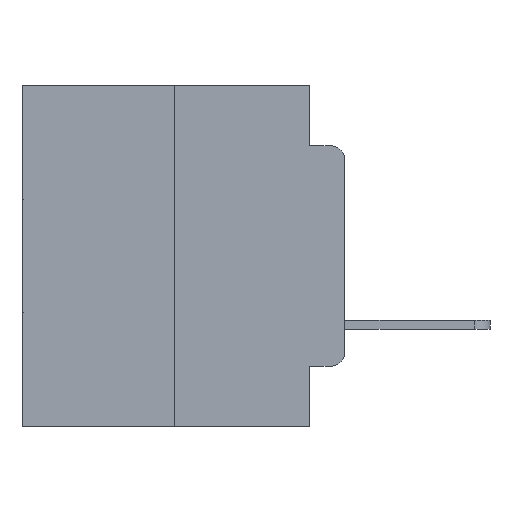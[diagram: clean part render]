
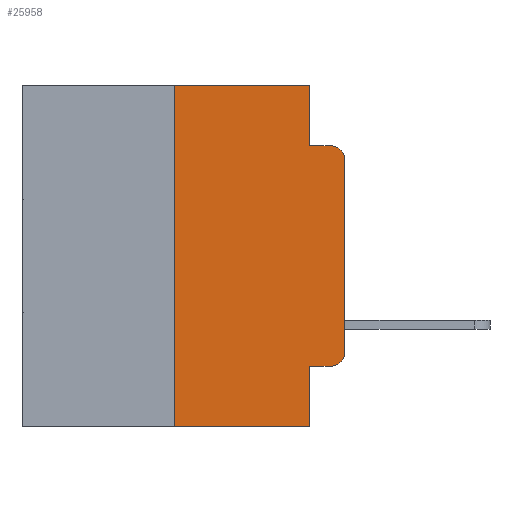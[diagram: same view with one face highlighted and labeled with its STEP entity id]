
A CAD part, left-side view. The second image highlights one B-rep face of the part: STEP entity #25958.
In plain terms, the highlighted planar face has unit normal (-1, 0, 0).
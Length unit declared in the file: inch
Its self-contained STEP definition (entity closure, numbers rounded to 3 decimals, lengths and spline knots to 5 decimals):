
#307 = EDGE_CURVE ( 'NONE', #18999, #11855, #12289, .T. ) ;
#1057 = DIRECTION ( 'NONE',  ( 0., 0., 1. ) ) ;
#2046 = EDGE_CURVE ( 'NONE', #11855, #27441, #28759, .T. ) ;
#3486 = ORIENTED_EDGE ( 'NONE', *, *, #28322, .T. ) ;
#3805 = CARTESIAN_POINT ( 'NONE',  ( 0., 0.473, 0. ) ) ;
#3833 = VERTEX_POINT ( 'NONE', #8795 ) ;
#4408 = LINE ( 'NONE', #28367, #21499 ) ;
#4472 = DIRECTION ( 'NONE',  ( 0., 0., -1. ) ) ;
#4509 = CIRCLE ( 'NONE', #9786, 0.02 ) ;
#4801 = ORIENTED_EDGE ( 'NONE', *, *, #6976, .T. ) ;
#5024 = CARTESIAN_POINT ( 'NONE',  ( 0., 0.25, 0. ) ) ;
#5761 = DIRECTION ( 'NONE',  ( -1., 0., 0. ) ) ;
#6005 = DIRECTION ( 'NONE',  ( 0., 0., -1. ) ) ;
#6073 = CARTESIAN_POINT ( 'NONE',  ( 0., 0.02, -0.3915 ) ) ;
#6218 = LINE ( 'NONE', #12638, #6965 ) ;
#6262 = VECTOR ( 'NONE', #6005, 39.37008 ) ;
#6522 = ORIENTED_EDGE ( 'NONE', *, *, #20888, .T. ) ;
#6965 = VECTOR ( 'NONE', #25672, 39.37008 ) ;
#6976 = EDGE_CURVE ( 'NONE', #25362, #27441, #17237, .T. ) ;
#7491 = FACE_OUTER_BOUND ( 'NONE', #21758, .T. ) ;
#7648 = VERTEX_POINT ( 'NONE', #16411 ) ;
#8306 = CARTESIAN_POINT ( 'NONE',  ( 0., 0.051, 0. ) ) ;
#8373 = DIRECTION ( 'NONE',  ( 0., 0., -1. ) ) ;
#8466 = EDGE_CURVE ( 'NONE', #13363, #25362, #14422, .T. ) ;
#8471 = VECTOR ( 'NONE', #1057, 39.37008 ) ;
#8795 = CARTESIAN_POINT ( 'NONE',  ( 0., 0.25, -0.5 ) ) ;
#8812 = ORIENTED_EDGE ( 'NONE', *, *, #13742, .F. ) ;
#9038 = CARTESIAN_POINT ( 'NONE',  ( 0., 0., -0.1085 ) ) ;
#9478 = VECTOR ( 'NONE', #16939, 39.37008 ) ;
#9786 = AXIS2_PLACEMENT_3D ( 'NONE', #6073, #21584, #8373 ) ;
#11038 = CARTESIAN_POINT ( 'NONE',  ( 0., 0.02, -0.4115 ) ) ;
#11855 = VERTEX_POINT ( 'NONE', #20120 ) ;
#12009 = CARTESIAN_POINT ( 'NONE',  ( 0., 0.02, -0.0885 ) ) ;
#12289 = LINE ( 'NONE', #8306, #6262 ) ;
#12303 = ORIENTED_EDGE ( 'NONE', *, *, #2046, .F. ) ;
#12527 = DIRECTION ( 'NONE',  ( 0., -1., 0. ) ) ;
#12638 = CARTESIAN_POINT ( 'NONE',  ( 0., 0.051, 0. ) ) ;
#12788 = ORIENTED_EDGE ( 'NONE', *, *, #27973, .F. ) ;
#13208 = VERTEX_POINT ( 'NONE', #22262 ) ;
#13363 = VERTEX_POINT ( 'NONE', #24741 ) ;
#13496 = CARTESIAN_POINT ( 'NONE',  ( 0., 0.473, 0. ) ) ;
#13694 = DIRECTION ( 'NONE',  ( 0., 0., 1. ) ) ;
#13742 = EDGE_CURVE ( 'NONE', #22176, #18999, #16349, .T. ) ;
#13881 = ORIENTED_EDGE ( 'NONE', *, *, #22297, .F. ) ;
#14422 = LINE ( 'NONE', #19356, #8471 ) ;
#15619 = ORIENTED_EDGE ( 'NONE', *, *, #8466, .T. ) ;
#15647 = VECTOR ( 'NONE', #21687, 39.37008 ) ;
#16349 = LINE ( 'NONE', #3805, #15647 ) ;
#16411 = CARTESIAN_POINT ( 'NONE',  ( 0., 0.051, -0.5 ) ) ;
#16425 = VECTOR ( 'NONE', #13694, 39.37008 ) ;
#16939 = DIRECTION ( 'NONE',  ( 0., -1., 0. ) ) ;
#16985 = CARTESIAN_POINT ( 'NONE',  ( 0., 0.051, 0. ) ) ;
#17038 = CARTESIAN_POINT ( 'NONE',  ( 0., 0.473, -0.5 ) ) ;
#17135 = VERTEX_POINT ( 'NONE', #11038 ) ;
#17237 = CIRCLE ( 'NONE', #24615, 0.02 ) ;
#17710 = DIRECTION ( 'NONE',  ( 0., -1., 0. ) ) ;
#17909 = DIRECTION ( 'NONE',  ( 1., 0., 0. ) ) ;
#18513 = LINE ( 'NONE', #20250, #16425 ) ;
#18999 = VERTEX_POINT ( 'NONE', #16985 ) ;
#19164 = CARTESIAN_POINT ( 'NONE',  ( 0., 0.02, -0.1085 ) ) ;
#19356 = CARTESIAN_POINT ( 'NONE',  ( 0., 0., 0. ) ) ;
#19433 = EDGE_CURVE ( 'NONE', #17135, #13363, #4509, .T. ) ;
#20054 = PLANE ( 'NONE',  #21831 ) ;
#20120 = CARTESIAN_POINT ( 'NONE',  ( 0., 0.051, -0.0885 ) ) ;
#20250 = CARTESIAN_POINT ( 'NONE',  ( 0., 0.25, 0. ) ) ;
#20888 = EDGE_CURVE ( 'NONE', #13208, #17135, #4408, .T. ) ;
#21304 = DIRECTION ( 'NONE',  ( 0., 0., -1. ) ) ;
#21499 = VECTOR ( 'NONE', #17710, 39.37008 ) ;
#21584 = DIRECTION ( 'NONE',  ( -1., 0., 0. ) ) ;
#21687 = DIRECTION ( 'NONE',  ( 0., -1., 0. ) ) ;
#21758 = EDGE_LOOP ( 'NONE', ( #15619, #4801, #12303, #21844, #8812, #12788, #3486, #13881, #6522, #24511 ) ) ;
#21831 = AXIS2_PLACEMENT_3D ( 'NONE', #13496, #17909, #4472 ) ;
#21844 = ORIENTED_EDGE ( 'NONE', *, *, #307, .F. ) ;
#22176 = VERTEX_POINT ( 'NONE', #5024 ) ;
#22262 = CARTESIAN_POINT ( 'NONE',  ( 0., 0.051, -0.4115 ) ) ;
#22297 = EDGE_CURVE ( 'NONE', #13208, #7648, #6218, .T. ) ;
#23175 = VECTOR ( 'NONE', #12527, 39.37008 ) ;
#24511 = ORIENTED_EDGE ( 'NONE', *, *, #19433, .T. ) ;
#24615 = AXIS2_PLACEMENT_3D ( 'NONE', #19164, #5761, #21304 ) ;
#24741 = CARTESIAN_POINT ( 'NONE',  ( 0., 0., -0.3915 ) ) ;
#25362 = VERTEX_POINT ( 'NONE', #9038 ) ;
#25402 = CARTESIAN_POINT ( 'NONE',  ( 0., 0.051, -0.0885 ) ) ;
#25542 = LINE ( 'NONE', #17038, #9478 ) ;
#25672 = DIRECTION ( 'NONE',  ( 0., 0., -1. ) ) ;
#25958 = ADVANCED_FACE ( 'NONE', ( #7491 ), #20054, .F. ) ;
#27441 = VERTEX_POINT ( 'NONE', #12009 ) ;
#27973 = EDGE_CURVE ( 'NONE', #3833, #22176, #18513, .T. ) ;
#28322 = EDGE_CURVE ( 'NONE', #3833, #7648, #25542, .T. ) ;
#28367 = CARTESIAN_POINT ( 'NONE',  ( 0., 0.051, -0.4115 ) ) ;
#28759 = LINE ( 'NONE', #25402, #23175 ) ;
